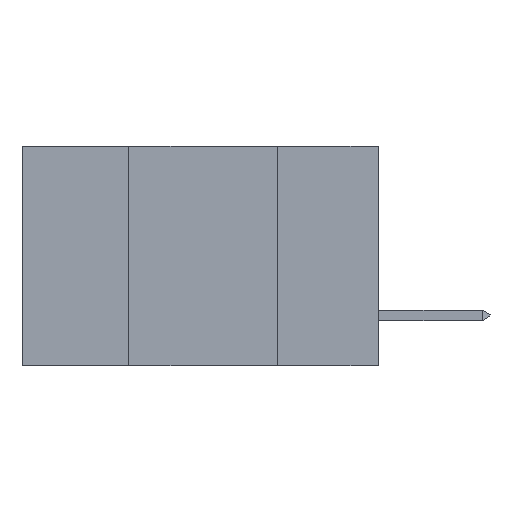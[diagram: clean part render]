
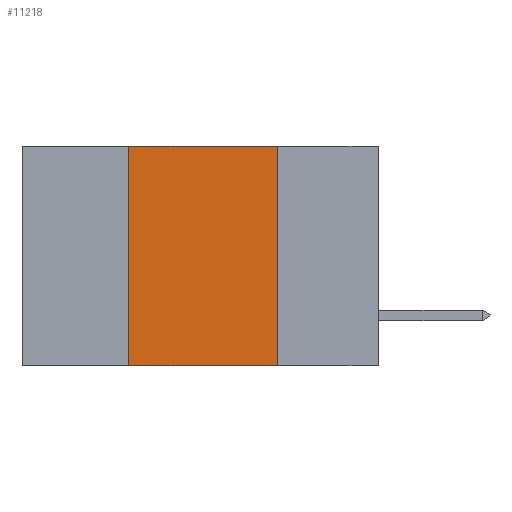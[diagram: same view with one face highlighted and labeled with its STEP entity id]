
A CAD part, left-side view. The second image highlights one B-rep face of the part: STEP entity #11218.
In plain terms, the highlighted planar face has unit normal (-1, 0, 0).
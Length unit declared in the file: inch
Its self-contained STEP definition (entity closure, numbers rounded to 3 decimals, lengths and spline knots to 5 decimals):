
#255 = VERTEX_POINT ( 'NONE', #7638 ) ;
#423 = VECTOR ( 'NONE', #7971, 39.37008 ) ;
#576 = LINE ( 'NONE', #816, #11230 ) ;
#816 = CARTESIAN_POINT ( 'NONE',  ( 0., 0.17, -0.37 ) ) ;
#858 = CARTESIAN_POINT ( 'NONE',  ( 0., 0.17, 0. ) ) ;
#1864 = LINE ( 'NONE', #6755, #12747 ) ;
#1885 = VERTEX_POINT ( 'NONE', #858 ) ;
#2097 = CARTESIAN_POINT ( 'NONE',  ( 0., 0.42, -0.37 ) ) ;
#2628 = CARTESIAN_POINT ( 'NONE',  ( 0., 0.6, 0. ) ) ;
#2642 = CARTESIAN_POINT ( 'NONE',  ( 0., 0.6, 0. ) ) ;
#3939 = DIRECTION ( 'NONE',  ( 1., 0., 0. ) ) ;
#4137 = EDGE_CURVE ( 'NONE', #6756, #1885, #14878, .T. ) ;
#4205 = EDGE_LOOP ( 'NONE', ( #8705, #15720, #6462, #15679 ) ) ;
#4264 = CARTESIAN_POINT ( 'NONE',  ( 0., 0.42, 0. ) ) ;
#5128 = PLANE ( 'NONE',  #9349 ) ;
#5704 = DIRECTION ( 'NONE',  ( 0., 0., -1. ) ) ;
#6462 = ORIENTED_EDGE ( 'NONE', *, *, #12226, .F. ) ;
#6755 = CARTESIAN_POINT ( 'NONE',  ( 0., 0.6, -0.37 ) ) ;
#6756 = VERTEX_POINT ( 'NONE', #4264 ) ;
#7473 = FACE_OUTER_BOUND ( 'NONE', #4205, .T. ) ;
#7534 = DIRECTION ( 'NONE',  ( 0., -1., 0. ) ) ;
#7638 = CARTESIAN_POINT ( 'NONE',  ( 0., 0.42, -0.37 ) ) ;
#7941 = EDGE_CURVE ( 'NONE', #1885, #9744, #576, .T. ) ;
#7971 = DIRECTION ( 'NONE',  ( 0., 0., 1. ) ) ;
#8094 = CARTESIAN_POINT ( 'NONE',  ( 0., 0.17, -0.37 ) ) ;
#8705 = ORIENTED_EDGE ( 'NONE', *, *, #7941, .F. ) ;
#9349 = AXIS2_PLACEMENT_3D ( 'NONE', #2642, #3939, #14965 ) ;
#9744 = VERTEX_POINT ( 'NONE', #8094 ) ;
#10544 = VECTOR ( 'NONE', #7534, 39.37008 ) ;
#11218 = ADVANCED_FACE ( 'NONE', ( #7473 ), #5128, .F. ) ;
#11230 = VECTOR ( 'NONE', #5704, 39.37008 ) ;
#12226 = EDGE_CURVE ( 'NONE', #255, #6756, #12986, .T. ) ;
#12747 = VECTOR ( 'NONE', #14114, 39.37008 ) ;
#12986 = LINE ( 'NONE', #2097, #423 ) ;
#14114 = DIRECTION ( 'NONE',  ( 0., -1., 0. ) ) ;
#14863 = EDGE_CURVE ( 'NONE', #255, #9744, #1864, .T. ) ;
#14878 = LINE ( 'NONE', #2628, #10544 ) ;
#14965 = DIRECTION ( 'NONE',  ( 0., 0., -1. ) ) ;
#15679 = ORIENTED_EDGE ( 'NONE', *, *, #14863, .T. ) ;
#15720 = ORIENTED_EDGE ( 'NONE', *, *, #4137, .F. ) ;
